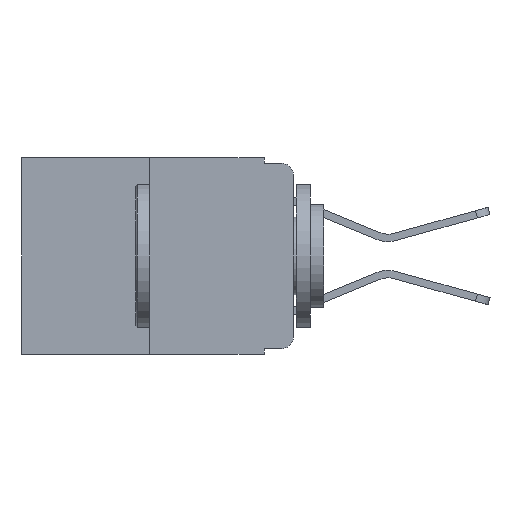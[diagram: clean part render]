
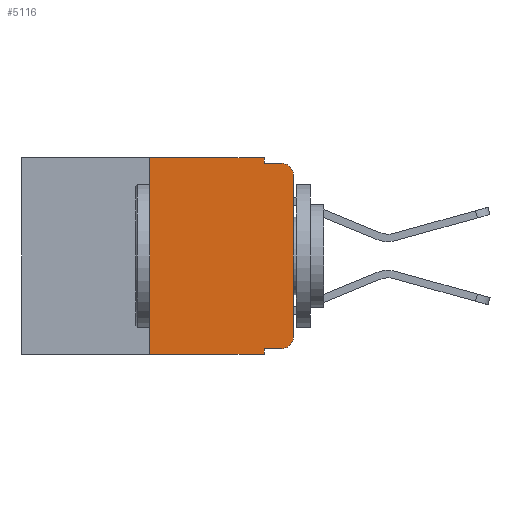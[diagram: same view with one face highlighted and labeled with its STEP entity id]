
A CAD part, left-side view. The second image highlights one B-rep face of the part: STEP entity #5116.
In plain terms, the highlighted planar face has unit normal (-1, 0, 0).
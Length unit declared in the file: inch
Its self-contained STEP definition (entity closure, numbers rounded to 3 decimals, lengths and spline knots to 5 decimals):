
#426 = CARTESIAN_POINT ( 'NONE',  ( 0., 0., 0. ) ) ;
#495 = VERTEX_POINT ( 'NONE', #10739 ) ;
#652 = EDGE_CURVE ( 'NONE', #2903, #7965, #3339, .T. ) ;
#734 = LINE ( 'NONE', #10386, #1702 ) ;
#925 = DIRECTION ( 'NONE',  ( 0., -1., 0. ) ) ;
#976 = CARTESIAN_POINT ( 'NONE',  ( 0., 0.02, -0.313 ) ) ;
#1365 = ORIENTED_EDGE ( 'NONE', *, *, #11383, .F. ) ;
#1554 = AXIS2_PLACEMENT_3D ( 'NONE', #13061, #6921, #6967 ) ;
#1560 = DIRECTION ( 'NONE',  ( 0., 0., 1. ) ) ;
#1678 = EDGE_CURVE ( 'NONE', #5630, #8175, #9214, .T. ) ;
#1694 = CARTESIAN_POINT ( 'NONE',  ( 0., 0.473, -0.343 ) ) ;
#1702 = VECTOR ( 'NONE', #7360, 39.37008 ) ;
#1741 = CARTESIAN_POINT ( 'NONE',  ( 0., 0.473, 0. ) ) ;
#1857 = CARTESIAN_POINT ( 'NONE',  ( 0., 0.051, -0.343 ) ) ;
#1886 = DIRECTION ( 'NONE',  ( 0., 0., -1. ) ) ;
#1915 = LINE ( 'NONE', #7022, #10508 ) ;
#2044 = VECTOR ( 'NONE', #12789, 39.37008 ) ;
#2046 = CARTESIAN_POINT ( 'NONE',  ( 0., 0.051, -0.01 ) ) ;
#2127 = ORIENTED_EDGE ( 'NONE', *, *, #8206, .T. ) ;
#2179 = AXIS2_PLACEMENT_3D ( 'NONE', #1741, #12197, #1886 ) ;
#2362 = VECTOR ( 'NONE', #12959, 39.37008 ) ;
#2880 = DIRECTION ( 'NONE',  ( 0., 0., 1. ) ) ;
#2903 = VERTEX_POINT ( 'NONE', #9631 ) ;
#3182 = LINE ( 'NONE', #426, #8915 ) ;
#3339 = LINE ( 'NONE', #2046, #9716 ) ;
#3437 = VERTEX_POINT ( 'NONE', #4627 ) ;
#3541 = ORIENTED_EDGE ( 'NONE', *, *, #10866, .T. ) ;
#3703 = VERTEX_POINT ( 'NONE', #11326 ) ;
#3727 = EDGE_CURVE ( 'NONE', #11008, #8175, #10106, .T. ) ;
#4012 = FACE_OUTER_BOUND ( 'NONE', #6547, .T. ) ;
#4091 = DIRECTION ( 'NONE',  ( 0., 0., -1. ) ) ;
#4534 = AXIS2_PLACEMENT_3D ( 'NONE', #976, #8163, #4091 ) ;
#4627 = CARTESIAN_POINT ( 'NONE',  ( 0., 0., -0.03 ) ) ;
#4777 = LINE ( 'NONE', #6303, #10829 ) ;
#5116 = ADVANCED_FACE ( 'NONE', ( #4012 ), #11936, .F. ) ;
#5211 = LINE ( 'NONE', #11762, #2044 ) ;
#5524 = ORIENTED_EDGE ( 'NONE', *, *, #6983, .F. ) ;
#5630 = VERTEX_POINT ( 'NONE', #7356 ) ;
#6097 = CARTESIAN_POINT ( 'NONE',  ( 0., 0.051, 0. ) ) ;
#6303 = CARTESIAN_POINT ( 'NONE',  ( 0., 0.473, 0. ) ) ;
#6547 = EDGE_LOOP ( 'NONE', ( #13044, #3541, #12367, #1365, #5524, #9521, #7595, #11063, #12953, #2127 ) ) ;
#6839 = CARTESIAN_POINT ( 'NONE',  ( 0., 0.25, 0. ) ) ;
#6921 = DIRECTION ( 'NONE',  ( -1., 0., 0. ) ) ;
#6967 = DIRECTION ( 'NONE',  ( 0., 0., -1. ) ) ;
#6983 = EDGE_CURVE ( 'NONE', #12998, #10200, #4777, .T. ) ;
#7022 = CARTESIAN_POINT ( 'NONE',  ( 0., 0.25, 0. ) ) ;
#7356 = CARTESIAN_POINT ( 'NONE',  ( 0., 0.25, -0.343 ) ) ;
#7360 = DIRECTION ( 'NONE',  ( 0., -1., 0. ) ) ;
#7567 = CARTESIAN_POINT ( 'NONE',  ( 0., 0.02, -0.01 ) ) ;
#7595 = ORIENTED_EDGE ( 'NONE', *, *, #1678, .T. ) ;
#7965 = VERTEX_POINT ( 'NONE', #7567 ) ;
#8163 = DIRECTION ( 'NONE',  ( -1., 0., 0. ) ) ;
#8175 = VERTEX_POINT ( 'NONE', #1857 ) ;
#8206 = EDGE_CURVE ( 'NONE', #495, #3703, #11290, .T. ) ;
#8915 = VECTOR ( 'NONE', #1560, 39.37008 ) ;
#9201 = CARTESIAN_POINT ( 'NONE',  ( 0., 0.051, -0.333 ) ) ;
#9214 = LINE ( 'NONE', #1694, #2362 ) ;
#9339 = CARTESIAN_POINT ( 'NONE',  ( 0., 0.051, 0. ) ) ;
#9521 = ORIENTED_EDGE ( 'NONE', *, *, #10213, .F. ) ;
#9631 = CARTESIAN_POINT ( 'NONE',  ( 0., 0.051, -0.01 ) ) ;
#9716 = VECTOR ( 'NONE', #12224, 39.37008 ) ;
#10038 = EDGE_CURVE ( 'NONE', #3703, #3437, #3182, .T. ) ;
#10106 = LINE ( 'NONE', #9339, #11070 ) ;
#10200 = VERTEX_POINT ( 'NONE', #6097 ) ;
#10213 = EDGE_CURVE ( 'NONE', #5630, #12998, #1915, .T. ) ;
#10386 = CARTESIAN_POINT ( 'NONE',  ( 0., 0.051, -0.333 ) ) ;
#10508 = VECTOR ( 'NONE', #2880, 39.37008 ) ;
#10739 = CARTESIAN_POINT ( 'NONE',  ( 0., 0.02, -0.333 ) ) ;
#10829 = VECTOR ( 'NONE', #925, 39.37008 ) ;
#10866 = EDGE_CURVE ( 'NONE', #3437, #7965, #11486, .T. ) ;
#11008 = VERTEX_POINT ( 'NONE', #9201 ) ;
#11063 = ORIENTED_EDGE ( 'NONE', *, *, #3727, .F. ) ;
#11070 = VECTOR ( 'NONE', #12353, 39.37008 ) ;
#11290 = CIRCLE ( 'NONE', #4534, 0.02 ) ;
#11326 = CARTESIAN_POINT ( 'NONE',  ( 0., 0., -0.313 ) ) ;
#11383 = EDGE_CURVE ( 'NONE', #10200, #2903, #5211, .T. ) ;
#11486 = CIRCLE ( 'NONE', #1554, 0.02 ) ;
#11710 = EDGE_CURVE ( 'NONE', #11008, #495, #734, .T. ) ;
#11762 = CARTESIAN_POINT ( 'NONE',  ( 0., 0.051, 0. ) ) ;
#11936 = PLANE ( 'NONE',  #2179 ) ;
#12197 = DIRECTION ( 'NONE',  ( 1., 0., 0. ) ) ;
#12224 = DIRECTION ( 'NONE',  ( 0., -1., 0. ) ) ;
#12353 = DIRECTION ( 'NONE',  ( 0., 0., -1. ) ) ;
#12367 = ORIENTED_EDGE ( 'NONE', *, *, #652, .F. ) ;
#12789 = DIRECTION ( 'NONE',  ( 0., 0., -1. ) ) ;
#12953 = ORIENTED_EDGE ( 'NONE', *, *, #11710, .T. ) ;
#12959 = DIRECTION ( 'NONE',  ( 0., -1., 0. ) ) ;
#12998 = VERTEX_POINT ( 'NONE', #6839 ) ;
#13044 = ORIENTED_EDGE ( 'NONE', *, *, #10038, .T. ) ;
#13061 = CARTESIAN_POINT ( 'NONE',  ( 0., 0.02, -0.03 ) ) ;
